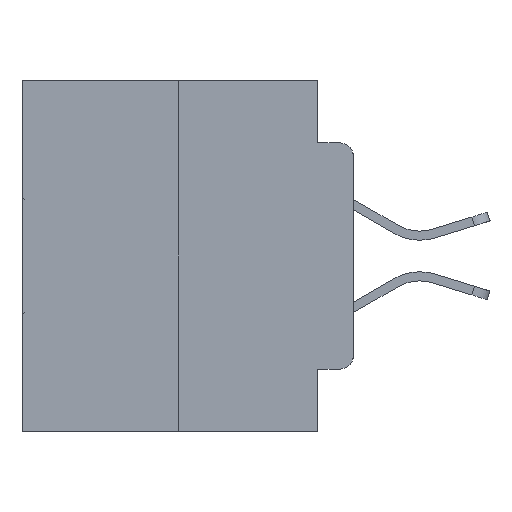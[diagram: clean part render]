
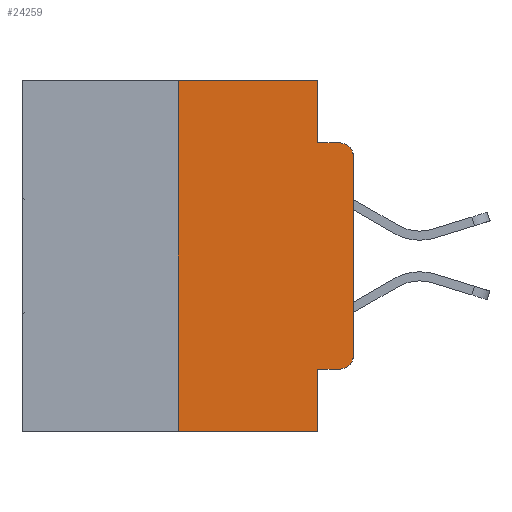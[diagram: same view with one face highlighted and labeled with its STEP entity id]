
A CAD part, left-side view. The second image highlights one B-rep face of the part: STEP entity #24259.
In plain terms, the highlighted planar face has unit normal (-1, 0, 0).
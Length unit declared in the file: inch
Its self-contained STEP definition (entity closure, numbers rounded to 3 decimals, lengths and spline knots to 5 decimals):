
#302 = CARTESIAN_POINT ( 'NONE',  ( 0., 0.25, -0.5 ) ) ;
#753 = DIRECTION ( 'NONE',  ( -1., 0., 0. ) ) ;
#781 = CARTESIAN_POINT ( 'NONE',  ( 0., 0.02, -0.3915 ) ) ;
#1084 = CARTESIAN_POINT ( 'NONE',  ( 0., 0.473, 0. ) ) ;
#1390 = CIRCLE ( 'NONE', #2502, 0.02 ) ;
#1795 = LINE ( 'NONE', #7133, #10918 ) ;
#2059 = LINE ( 'NONE', #29849, #9002 ) ;
#2218 = CARTESIAN_POINT ( 'NONE',  ( 0., 0., -0.3915 ) ) ;
#2502 = AXIS2_PLACEMENT_3D ( 'NONE', #781, #19215, #19011 ) ;
#3414 = CARTESIAN_POINT ( 'NONE',  ( 0., 0., 0. ) ) ;
#4687 = VECTOR ( 'NONE', #9942, 39.37008 ) ;
#5220 = ORIENTED_EDGE ( 'NONE', *, *, #14979, .F. ) ;
#6326 = CARTESIAN_POINT ( 'NONE',  ( 0., 0.473, 0. ) ) ;
#6492 = EDGE_CURVE ( 'NONE', #14447, #13488, #1795, .T. ) ;
#6504 = CARTESIAN_POINT ( 'NONE',  ( 0., 0.02, -0.4115 ) ) ;
#7133 = CARTESIAN_POINT ( 'NONE',  ( 0., 0.051, -0.4115 ) ) ;
#7211 = ORIENTED_EDGE ( 'NONE', *, *, #15761, .T. ) ;
#7316 = ORIENTED_EDGE ( 'NONE', *, *, #6492, .T. ) ;
#7376 = VERTEX_POINT ( 'NONE', #23671 ) ;
#7436 = CARTESIAN_POINT ( 'NONE',  ( 0., 0.473, -0.5 ) ) ;
#7943 = CARTESIAN_POINT ( 'NONE',  ( 0., 0.051, -0.4115 ) ) ;
#7977 = LINE ( 'NONE', #16174, #18543 ) ;
#8287 = VECTOR ( 'NONE', #17481, 39.37008 ) ;
#9002 = VECTOR ( 'NONE', #13709, 39.37008 ) ;
#9037 = LINE ( 'NONE', #1084, #8287 ) ;
#9598 = CIRCLE ( 'NONE', #10945, 0.02 ) ;
#9782 = DIRECTION ( 'NONE',  ( 0., -1., 0. ) ) ;
#9942 = DIRECTION ( 'NONE',  ( 0., -1., 0. ) ) ;
#10207 = EDGE_CURVE ( 'NONE', #14447, #7376, #2059, .T. ) ;
#10918 = VECTOR ( 'NONE', #27947, 39.37008 ) ;
#10945 = AXIS2_PLACEMENT_3D ( 'NONE', #12256, #753, #23990 ) ;
#11019 = DIRECTION ( 'NONE',  ( 1., 0., 0. ) ) ;
#11517 = VERTEX_POINT ( 'NONE', #12026 ) ;
#11828 = FACE_OUTER_BOUND ( 'NONE', #16082, .T. ) ;
#12026 = CARTESIAN_POINT ( 'NONE',  ( 0., 0.25, 0. ) ) ;
#12256 = CARTESIAN_POINT ( 'NONE',  ( 0., 0.02, -0.1085 ) ) ;
#12270 = ORIENTED_EDGE ( 'NONE', *, *, #10207, .F. ) ;
#13026 = LINE ( 'NONE', #20847, #23241 ) ;
#13488 = VERTEX_POINT ( 'NONE', #6504 ) ;
#13507 = VECTOR ( 'NONE', #9782, 39.37008 ) ;
#13654 = ORIENTED_EDGE ( 'NONE', *, *, #22947, .T. ) ;
#13709 = DIRECTION ( 'NONE',  ( 0., 0., -1. ) ) ;
#14299 = VERTEX_POINT ( 'NONE', #302 ) ;
#14390 = EDGE_CURVE ( 'NONE', #14299, #7376, #22238, .T. ) ;
#14423 = DIRECTION ( 'NONE',  ( 0., 0., 1. ) ) ;
#14447 = VERTEX_POINT ( 'NONE', #7943 ) ;
#14940 = VERTEX_POINT ( 'NONE', #2218 ) ;
#14974 = EDGE_CURVE ( 'NONE', #14299, #11517, #7977, .T. ) ;
#14979 = EDGE_CURVE ( 'NONE', #16144, #28813, #25852, .T. ) ;
#15761 = EDGE_CURVE ( 'NONE', #13488, #14940, #1390, .T. ) ;
#16082 = EDGE_LOOP ( 'NONE', ( #13654, #16350, #5220, #17366, #17291, #22954, #20364, #12270, #7316, #7211 ) ) ;
#16144 = VERTEX_POINT ( 'NONE', #18494 ) ;
#16174 = CARTESIAN_POINT ( 'NONE',  ( 0., 0.25, 0. ) ) ;
#16350 = ORIENTED_EDGE ( 'NONE', *, *, #18358, .T. ) ;
#16664 = CARTESIAN_POINT ( 'NONE',  ( 0., 0.051, -0.0885 ) ) ;
#17291 = ORIENTED_EDGE ( 'NONE', *, *, #22959, .F. ) ;
#17366 = ORIENTED_EDGE ( 'NONE', *, *, #27472, .F. ) ;
#17481 = DIRECTION ( 'NONE',  ( 0., -1., 0. ) ) ;
#18120 = VECTOR ( 'NONE', #26479, 39.37008 ) ;
#18358 = EDGE_CURVE ( 'NONE', #29055, #28813, #9598, .T. ) ;
#18494 = CARTESIAN_POINT ( 'NONE',  ( 0., 0.051, -0.0885 ) ) ;
#18543 = VECTOR ( 'NONE', #14423, 39.37008 ) ;
#19011 = DIRECTION ( 'NONE',  ( 0., 0., -1. ) ) ;
#19029 = CARTESIAN_POINT ( 'NONE',  ( 0., 0.02, -0.0885 ) ) ;
#19215 = DIRECTION ( 'NONE',  ( -1., 0., 0. ) ) ;
#20317 = LINE ( 'NONE', #3414, #18120 ) ;
#20364 = ORIENTED_EDGE ( 'NONE', *, *, #14390, .T. ) ;
#20847 = CARTESIAN_POINT ( 'NONE',  ( 0., 0.051, 0. ) ) ;
#21781 = AXIS2_PLACEMENT_3D ( 'NONE', #6326, #11019, #29894 ) ;
#22238 = LINE ( 'NONE', #7436, #13507 ) ;
#22947 = EDGE_CURVE ( 'NONE', #14940, #29055, #20317, .T. ) ;
#22954 = ORIENTED_EDGE ( 'NONE', *, *, #14974, .F. ) ;
#22959 = EDGE_CURVE ( 'NONE', #11517, #23652, #9037, .T. ) ;
#23241 = VECTOR ( 'NONE', #24104, 39.37008 ) ;
#23652 = VERTEX_POINT ( 'NONE', #29524 ) ;
#23671 = CARTESIAN_POINT ( 'NONE',  ( 0., 0.051, -0.5 ) ) ;
#23990 = DIRECTION ( 'NONE',  ( 0., 0., -1. ) ) ;
#24104 = DIRECTION ( 'NONE',  ( 0., 0., -1. ) ) ;
#24259 = ADVANCED_FACE ( 'NONE', ( #11828 ), #25176, .F. ) ;
#24543 = CARTESIAN_POINT ( 'NONE',  ( 0., 0., -0.1085 ) ) ;
#25176 = PLANE ( 'NONE',  #21781 ) ;
#25852 = LINE ( 'NONE', #16664, #4687 ) ;
#26479 = DIRECTION ( 'NONE',  ( 0., 0., 1. ) ) ;
#27472 = EDGE_CURVE ( 'NONE', #23652, #16144, #13026, .T. ) ;
#27947 = DIRECTION ( 'NONE',  ( 0., -1., 0. ) ) ;
#28813 = VERTEX_POINT ( 'NONE', #19029 ) ;
#29055 = VERTEX_POINT ( 'NONE', #24543 ) ;
#29524 = CARTESIAN_POINT ( 'NONE',  ( 0., 0.051, 0. ) ) ;
#29849 = CARTESIAN_POINT ( 'NONE',  ( 0., 0.051, 0. ) ) ;
#29894 = DIRECTION ( 'NONE',  ( 0., 0., -1. ) ) ;
